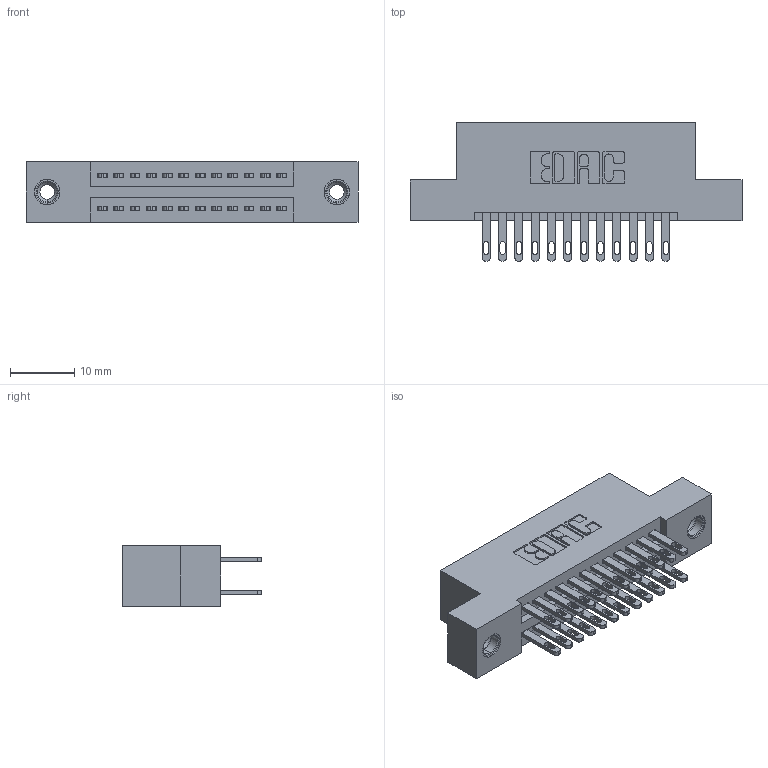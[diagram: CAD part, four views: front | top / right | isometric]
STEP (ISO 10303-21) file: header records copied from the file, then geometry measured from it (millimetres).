
FILE_DESCRIPTION (( 'STEP AP203' ), '1' );
FILE_NAME ('345-024-500-208.STEP', '2018-08-21T04:22:07', ( '' ), ( '' ), 'SwSTEP 2.0', 'SolidWorks 2016', '' );
FILE_SCHEMA (( 'CONFIG_CONTROL_DESIGN' ));
Length unit declared in the file: inch
Products named in the file (4): 345-292-001_345-293-100; 345-250-001_345-250-003-102; 345-024-500-208; 345 Part_Flush Mounting Lugs - 0.156 Dia-TI
Assembly tree (27 placements, depth 2):
  345-024-500-208
    345 Part_Flush Mounting Lugs - 0.156 Dia-TI
    345-292-001_345-293-100  x24
    345-250-001_345-250-003-102  x2
Bounding box: 51.69 x 21.51 x 9.4 mm (x, y, z)
Volume: 4809.5 mm3; surface area: 6786.4 mm2
Topology: 27 solids, 27 shells, 1290 faces, 3861 edges, 2566 vertices
Faces by surface type: plane 760, cylinder 514, cone 12, torus 4
Entity records: 14570 total; most frequent: CARTESIAN_POINT 2451, ORIENTED_EDGE 2378, DIRECTION 2227, EDGE_CURVE 1189, VECTOR 985, LINE 985, VERTEX_POINT 788, AXIS2_PLACEMENT_3D 621
